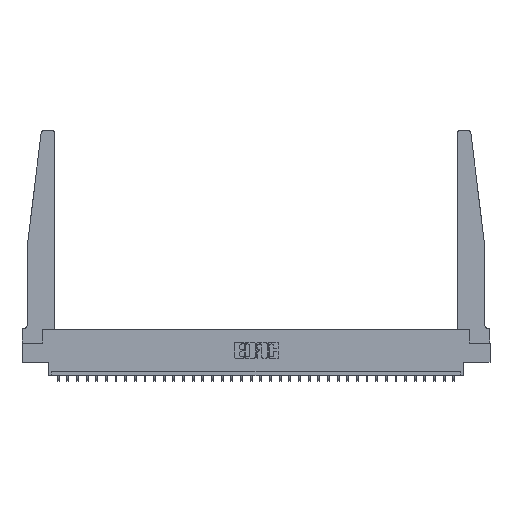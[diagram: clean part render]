
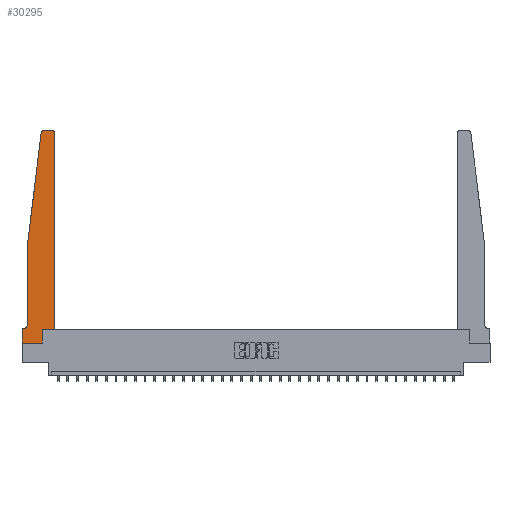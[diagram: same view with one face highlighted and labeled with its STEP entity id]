
A CAD part, top view. The second image highlights one B-rep face of the part: STEP entity #30295.
In plain terms, the highlighted planar face has unit normal (0, 0, 1).
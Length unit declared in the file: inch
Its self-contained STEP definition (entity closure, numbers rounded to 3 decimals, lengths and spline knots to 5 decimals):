
#91 = DIRECTION ( 'NONE',  ( 0., 0., 1. ) ) ;
#1274 = EDGE_CURVE ( 'NONE', #6467, #30012, #12233, .T. ) ;
#1732 = LINE ( 'NONE', #11426, #30911 ) ;
#1811 = EDGE_CURVE ( 'NONE', #1890, #13134, #15798, .T. ) ;
#1890 = VERTEX_POINT ( 'NONE', #20583 ) ;
#2128 = DIRECTION ( 'NONE',  ( -0.122, -0.992, 0. ) ) ;
#2195 = CARTESIAN_POINT ( 'NONE',  ( 0., 0.1875, 0.37 ) ) ;
#2245 = CARTESIAN_POINT ( 'NONE',  ( 0.015, 0.1875, 0.37 ) ) ;
#2592 = VECTOR ( 'NONE', #26431, 39.37008 ) ;
#3656 = ORIENTED_EDGE ( 'NONE', *, *, #1811, .T. ) ;
#3763 = ORIENTED_EDGE ( 'NONE', *, *, #6539, .T. ) ;
#4105 = CARTESIAN_POINT ( 'NONE',  ( 0.395, 2.75, 0.37 ) ) ;
#4577 = EDGE_LOOP ( 'NONE', ( #24315, #21787, #20709, #3656, #24237, #14461, #3763, #7630, #29037, #19109, #8698, #17709 ) ) ;
#4639 = VERTEX_POINT ( 'NONE', #4950 ) ;
#4714 = EDGE_CURVE ( 'NONE', #8666, #6534, #22655, .T. ) ;
#4746 = VECTOR ( 'NONE', #7834, 39.37008 ) ;
#4950 = CARTESIAN_POINT ( 'NONE',  ( 0.2605, 0.18, 0.37 ) ) ;
#5197 = CARTESIAN_POINT ( 'NONE',  ( 0., 0., 0.37 ) ) ;
#5807 = VECTOR ( 'NONE', #2128, 39.37008 ) ;
#6467 = VERTEX_POINT ( 'NONE', #4105 ) ;
#6507 = VERTEX_POINT ( 'NONE', #20690 ) ;
#6534 = VERTEX_POINT ( 'NONE', #2195 ) ;
#6539 = EDGE_CURVE ( 'NONE', #6534, #17273, #16692, .T. ) ;
#7347 = CARTESIAN_POINT ( 'NONE',  ( 0.065, 1.25, 0.37 ) ) ;
#7548 = DIRECTION ( 'NONE',  ( 1., 0., 0. ) ) ;
#7630 = ORIENTED_EDGE ( 'NONE', *, *, #29900, .T. ) ;
#7794 = FACE_OUTER_BOUND ( 'NONE', #4577, .T. ) ;
#7834 = DIRECTION ( 'NONE',  ( 1., 0., 0. ) ) ;
#8268 = DIRECTION ( 'NONE',  ( -1., 0., 0. ) ) ;
#8427 = CARTESIAN_POINT ( 'NONE',  ( 0.065, 0.1875, 0.37 ) ) ;
#8666 = VERTEX_POINT ( 'NONE', #2245 ) ;
#8698 = ORIENTED_EDGE ( 'NONE', *, *, #27678, .T. ) ;
#8974 = DIRECTION ( 'NONE',  ( 1., 0., 0. ) ) ;
#9567 = LINE ( 'NONE', #12296, #15641 ) ;
#9660 = CARTESIAN_POINT ( 'NONE',  ( 0.25, 2.75, 0.37 ) ) ;
#10008 = AXIS2_PLACEMENT_3D ( 'NONE', #30439, #20401, #17852 ) ;
#10338 = LINE ( 'NONE', #21845, #12888 ) ;
#10684 = CARTESIAN_POINT ( 'NONE',  ( 0., 0.1875, 0.37 ) ) ;
#11065 = CARTESIAN_POINT ( 'NONE',  ( 0.065, 0.2375, 0.37 ) ) ;
#11148 = DIRECTION ( 'NONE',  ( 1., 0., 0. ) ) ;
#11426 = CARTESIAN_POINT ( 'NONE',  ( 0.425, 0.18, 0.37 ) ) ;
#11633 = EDGE_CURVE ( 'NONE', #30012, #21959, #26736, .T. ) ;
#12233 = LINE ( 'NONE', #9660, #13153 ) ;
#12296 = CARTESIAN_POINT ( 'NONE',  ( 0.2605, 0.18, 0.37 ) ) ;
#12599 = AXIS2_PLACEMENT_3D ( 'NONE', #23199, #18865, #8974 ) ;
#12888 = VECTOR ( 'NONE', #19598, 39.37008 ) ;
#12995 = AXIS2_PLACEMENT_3D ( 'NONE', #19830, #91, #7548 ) ;
#13095 = CARTESIAN_POINT ( 'NONE',  ( 0.065, 1.25, 0.37 ) ) ;
#13134 = VERTEX_POINT ( 'NONE', #11065 ) ;
#13153 = VECTOR ( 'NONE', #29129, 39.37008 ) ;
#13422 = CARTESIAN_POINT ( 'NONE',  ( 0.27653, 2.75, 0.37 ) ) ;
#14183 = VERTEX_POINT ( 'NONE', #18784 ) ;
#14461 = ORIENTED_EDGE ( 'NONE', *, *, #4714, .T. ) ;
#14528 = VERTEX_POINT ( 'NONE', #30831 ) ;
#15641 = VECTOR ( 'NONE', #28892, 39.37008 ) ;
#15798 = LINE ( 'NONE', #13095, #16731 ) ;
#16367 = DIRECTION ( 'NONE',  ( 1., 0., 0. ) ) ;
#16692 = LINE ( 'NONE', #5197, #2592 ) ;
#16731 = VECTOR ( 'NONE', #18188, 39.37008 ) ;
#16928 = EDGE_CURVE ( 'NONE', #21959, #1890, #26508, .T. ) ;
#17273 = VERTEX_POINT ( 'NONE', #30157 ) ;
#17709 = ORIENTED_EDGE ( 'NONE', *, *, #20652, .T. ) ;
#17852 = DIRECTION ( 'NONE',  ( -1., 0., 0. ) ) ;
#18188 = DIRECTION ( 'NONE',  ( 0., -1., 0. ) ) ;
#18320 = PLANE ( 'NONE',  #19022 ) ;
#18784 = CARTESIAN_POINT ( 'NONE',  ( 0.2605, 0., 0.37 ) ) ;
#18865 = DIRECTION ( 'NONE',  ( 0., 0., 1. ) ) ;
#19022 = AXIS2_PLACEMENT_3D ( 'NONE', #10684, #28059, #11148 ) ;
#19109 = ORIENTED_EDGE ( 'NONE', *, *, #20253, .T. ) ;
#19494 = CARTESIAN_POINT ( 'NONE',  ( 0.24675, 2.72367, 0.37 ) ) ;
#19591 = EDGE_CURVE ( 'NONE', #13134, #8666, #23251, .T. ) ;
#19598 = DIRECTION ( 'NONE',  ( 0., 1., 0. ) ) ;
#19830 = CARTESIAN_POINT ( 'NONE',  ( 0.27653, 2.72, 0.37 ) ) ;
#19961 = LINE ( 'NONE', #29705, #4746 ) ;
#20253 = EDGE_CURVE ( 'NONE', #4639, #14528, #1732, .T. ) ;
#20401 = DIRECTION ( 'NONE',  ( 0., 0., -1. ) ) ;
#20583 = CARTESIAN_POINT ( 'NONE',  ( 0.065, 1.25, 0.37 ) ) ;
#20652 = EDGE_CURVE ( 'NONE', #6507, #6467, #30410, .T. ) ;
#20690 = CARTESIAN_POINT ( 'NONE',  ( 0.425, 2.72, 0.37 ) ) ;
#20709 = ORIENTED_EDGE ( 'NONE', *, *, #16928, .T. ) ;
#21787 = ORIENTED_EDGE ( 'NONE', *, *, #11633, .T. ) ;
#21845 = CARTESIAN_POINT ( 'NONE',  ( 0.425, 0.18, 0.37 ) ) ;
#21959 = VERTEX_POINT ( 'NONE', #19494 ) ;
#22245 = EDGE_CURVE ( 'NONE', #14183, #4639, #9567, .T. ) ;
#22655 = LINE ( 'NONE', #8427, #28899 ) ;
#23199 = CARTESIAN_POINT ( 'NONE',  ( 0.395, 2.72, 0.37 ) ) ;
#23251 = CIRCLE ( 'NONE', #10008, 0.05 ) ;
#24237 = ORIENTED_EDGE ( 'NONE', *, *, #19591, .T. ) ;
#24315 = ORIENTED_EDGE ( 'NONE', *, *, #1274, .T. ) ;
#26431 = DIRECTION ( 'NONE',  ( 0., -1., 0. ) ) ;
#26508 = LINE ( 'NONE', #7347, #5807 ) ;
#26736 = CIRCLE ( 'NONE', #12995, 0.03 ) ;
#27678 = EDGE_CURVE ( 'NONE', #14528, #6507, #10338, .T. ) ;
#28059 = DIRECTION ( 'NONE',  ( 0., 0., 1. ) ) ;
#28892 = DIRECTION ( 'NONE',  ( 0., 1., 0. ) ) ;
#28899 = VECTOR ( 'NONE', #8268, 39.37008 ) ;
#29037 = ORIENTED_EDGE ( 'NONE', *, *, #22245, .T. ) ;
#29129 = DIRECTION ( 'NONE',  ( -1., 0., 0. ) ) ;
#29705 = CARTESIAN_POINT ( 'NONE',  ( 0., 0., 0.37 ) ) ;
#29900 = EDGE_CURVE ( 'NONE', #17273, #14183, #19961, .T. ) ;
#30012 = VERTEX_POINT ( 'NONE', #13422 ) ;
#30157 = CARTESIAN_POINT ( 'NONE',  ( 0., 0., 0.37 ) ) ;
#30295 = ADVANCED_FACE ( 'NONE', ( #7794 ), #18320, .T. ) ;
#30410 = CIRCLE ( 'NONE', #12599, 0.03 ) ;
#30439 = CARTESIAN_POINT ( 'NONE',  ( 0.015, 0.2375, 0.37 ) ) ;
#30831 = CARTESIAN_POINT ( 'NONE',  ( 0.425, 0.18, 0.37 ) ) ;
#30911 = VECTOR ( 'NONE', #16367, 39.37008 ) ;
